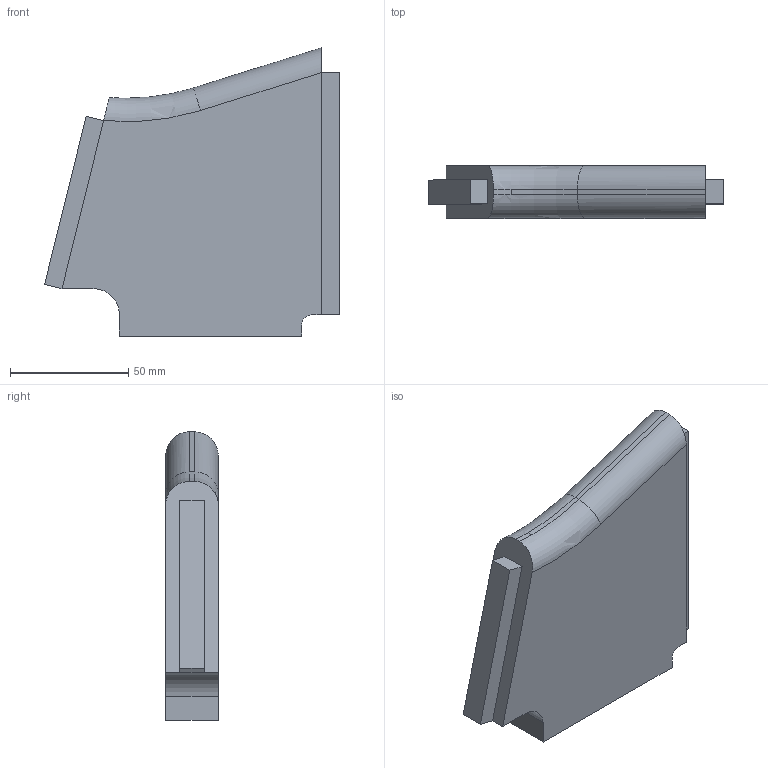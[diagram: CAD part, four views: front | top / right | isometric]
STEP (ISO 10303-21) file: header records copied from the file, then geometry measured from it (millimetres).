
FILE_DESCRIPTION (( 'STEP AP214' ), '1' );
FILE_NAME ('hydrastockx2.STEP', '2013-07-04T02:27:31', ( '' ), ( '' ), 'SwSTEP 2.0', 'SolidWorks 2012', '' );
FILE_SCHEMA (( 'AUTOMOTIVE_DESIGN' ));
Length unit declared in the file: inch
Products named in the file (1): hydrastockx2
Bounding box: 124.71 x 22.24 x 121.94 mm (x, y, z)
Volume: 241831 mm3; surface area: 32349.9 mm2
Topology: 1 solids, 1 shells, 27 faces, 71 edges, 46 vertices
Faces by surface type: plane 19, cylinder 6, torus 2
Entity records: 906 total; most frequent: CARTESIAN_POINT 196, ORIENTED_EDGE 142, DIRECTION 135, EDGE_CURVE 71, LINE 55, VECTOR 55, VERTEX_POINT 46, AXIS2_PLACEMENT_3D 40
